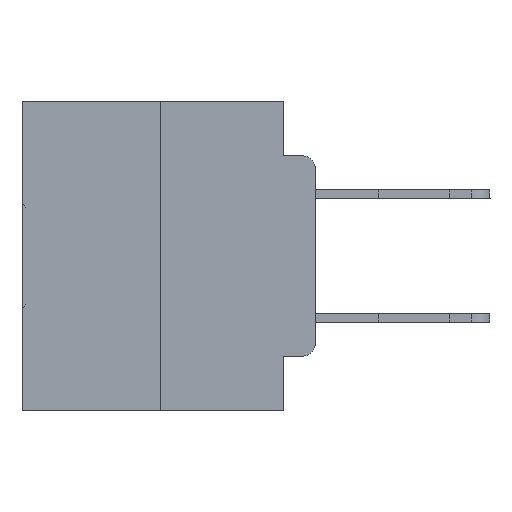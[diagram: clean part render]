
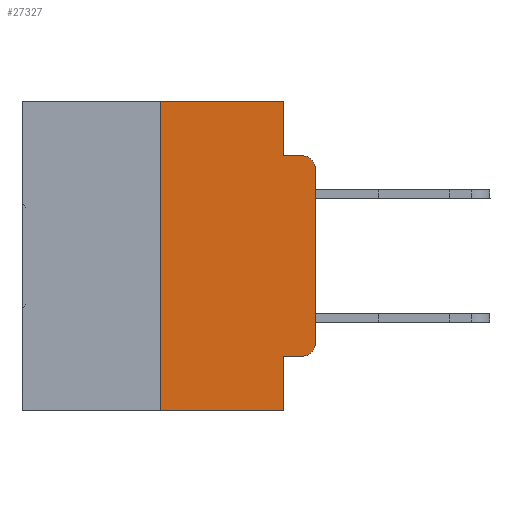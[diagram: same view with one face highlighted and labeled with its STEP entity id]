
A CAD part, left-side view. The second image highlights one B-rep face of the part: STEP entity #27327.
In plain terms, the highlighted planar face has unit normal (-1, 0, 0).
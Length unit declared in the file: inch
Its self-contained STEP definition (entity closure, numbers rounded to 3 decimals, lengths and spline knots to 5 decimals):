
#2213 = CARTESIAN_POINT ( 'NONE',  ( 0., 0.25, 0. ) ) ;
#2262 = VERTEX_POINT ( 'NONE', #5956 ) ;
#2728 = CARTESIAN_POINT ( 'NONE',  ( 0., 0.051, 0. ) ) ;
#3521 = VERTEX_POINT ( 'NONE', #10878 ) ;
#3592 = VERTEX_POINT ( 'NONE', #6604 ) ;
#4012 = ORIENTED_EDGE ( 'NONE', *, *, #5354, .F. ) ;
#4303 = DIRECTION ( 'NONE',  ( 0., -1., 0. ) ) ;
#4450 = VECTOR ( 'NONE', #5321, 39.37008 ) ;
#4704 = CARTESIAN_POINT ( 'NONE',  ( 0., 0.051, -0.0885 ) ) ;
#4944 = CARTESIAN_POINT ( 'NONE',  ( 0., 0.02, -0.0885 ) ) ;
#5089 = VERTEX_POINT ( 'NONE', #11363 ) ;
#5298 = EDGE_CURVE ( 'NONE', #19324, #2262, #17983, .T. ) ;
#5321 = DIRECTION ( 'NONE',  ( 0., 0., -1. ) ) ;
#5354 = EDGE_CURVE ( 'NONE', #12511, #17795, #28967, .T. ) ;
#5647 = PLANE ( 'NONE',  #28831 ) ;
#5956 = CARTESIAN_POINT ( 'NONE',  ( 0., 0.051, -0.5 ) ) ;
#6230 = ORIENTED_EDGE ( 'NONE', *, *, #12284, .F. ) ;
#6259 = ORIENTED_EDGE ( 'NONE', *, *, #5298, .T. ) ;
#6604 = CARTESIAN_POINT ( 'NONE',  ( 0., 0.02, -0.4115 ) ) ;
#6628 = DIRECTION ( 'NONE',  ( -1., 0., 0. ) ) ;
#6842 = VERTEX_POINT ( 'NONE', #19557 ) ;
#7045 = EDGE_CURVE ( 'NONE', #5089, #12511, #17865, .T. ) ;
#7647 = VECTOR ( 'NONE', #18603, 39.37008 ) ;
#8084 = VECTOR ( 'NONE', #4303, 39.37008 ) ;
#8150 = DIRECTION ( 'NONE',  ( 0., 0., -1. ) ) ;
#10613 = EDGE_LOOP ( 'NONE', ( #29082, #21397, #4012, #15840, #6230, #30624, #6259, #30481, #12213, #14582 ) ) ;
#10704 = VECTOR ( 'NONE', #24773, 39.37008 ) ;
#10878 = CARTESIAN_POINT ( 'NONE',  ( 0., 0., -0.1085 ) ) ;
#11234 = LINE ( 'NONE', #31539, #12017 ) ;
#11363 = CARTESIAN_POINT ( 'NONE',  ( 0., 0.051, 0. ) ) ;
#12017 = VECTOR ( 'NONE', #19038, 39.37008 ) ;
#12142 = EDGE_CURVE ( 'NONE', #6842, #2262, #21060, .T. ) ;
#12213 = ORIENTED_EDGE ( 'NONE', *, *, #20557, .T. ) ;
#12284 = EDGE_CURVE ( 'NONE', #32064, #5089, #11234, .T. ) ;
#12376 = DIRECTION ( 'NONE',  ( 0., -1., 0. ) ) ;
#12511 = VERTEX_POINT ( 'NONE', #4704 ) ;
#12925 = CARTESIAN_POINT ( 'NONE',  ( 0., 0.25, 0. ) ) ;
#13269 = LINE ( 'NONE', #30230, #25851 ) ;
#13841 = EDGE_CURVE ( 'NONE', #19324, #32064, #16252, .T. ) ;
#14211 = CIRCLE ( 'NONE', #20802, 0.02 ) ;
#14582 = ORIENTED_EDGE ( 'NONE', *, *, #15503, .T. ) ;
#14964 = DIRECTION ( 'NONE',  ( -1., 0., 0. ) ) ;
#15434 = DIRECTION ( 'NONE',  ( 0., 0., 1. ) ) ;
#15503 = EDGE_CURVE ( 'NONE', #3592, #26535, #14211, .T. ) ;
#15840 = ORIENTED_EDGE ( 'NONE', *, *, #7045, .F. ) ;
#16053 = CARTESIAN_POINT ( 'NONE',  ( 0., 0.051, 0. ) ) ;
#16252 = LINE ( 'NONE', #12925, #28836 ) ;
#17184 = VECTOR ( 'NONE', #12376, 39.37008 ) ;
#17795 = VERTEX_POINT ( 'NONE', #4944 ) ;
#17821 = EDGE_CURVE ( 'NONE', #26535, #3521, #13269, .T. ) ;
#17865 = LINE ( 'NONE', #2728, #4450 ) ;
#17983 = LINE ( 'NONE', #29927, #17184 ) ;
#18099 = CARTESIAN_POINT ( 'NONE',  ( 0., 0.473, 0. ) ) ;
#18603 = DIRECTION ( 'NONE',  ( 0., 0., -1. ) ) ;
#18857 = FACE_OUTER_BOUND ( 'NONE', #10613, .T. ) ;
#19038 = DIRECTION ( 'NONE',  ( 0., -1., 0. ) ) ;
#19324 = VERTEX_POINT ( 'NONE', #26350 ) ;
#19557 = CARTESIAN_POINT ( 'NONE',  ( 0., 0.051, -0.4115 ) ) ;
#20557 = EDGE_CURVE ( 'NONE', #6842, #3592, #30727, .T. ) ;
#20802 = AXIS2_PLACEMENT_3D ( 'NONE', #29999, #14964, #32491 ) ;
#21060 = LINE ( 'NONE', #16053, #7647 ) ;
#21397 = ORIENTED_EDGE ( 'NONE', *, *, #22882, .T. ) ;
#21741 = CARTESIAN_POINT ( 'NONE',  ( 0., 0.02, -0.1085 ) ) ;
#22209 = CARTESIAN_POINT ( 'NONE',  ( 0., 0.051, -0.4115 ) ) ;
#22795 = CIRCLE ( 'NONE', #31477, 0.02 ) ;
#22882 = EDGE_CURVE ( 'NONE', #3521, #17795, #22795, .T. ) ;
#23290 = DIRECTION ( 'NONE',  ( 1., 0., 0. ) ) ;
#24300 = DIRECTION ( 'NONE',  ( 0., 0., -1. ) ) ;
#24773 = DIRECTION ( 'NONE',  ( 0., -1., 0. ) ) ;
#25851 = VECTOR ( 'NONE', #32730, 39.37008 ) ;
#26350 = CARTESIAN_POINT ( 'NONE',  ( 0., 0.25, -0.5 ) ) ;
#26535 = VERTEX_POINT ( 'NONE', #29905 ) ;
#26990 = CARTESIAN_POINT ( 'NONE',  ( 0., 0.051, -0.0885 ) ) ;
#27327 = ADVANCED_FACE ( 'NONE', ( #18857 ), #5647, .F. ) ;
#28831 = AXIS2_PLACEMENT_3D ( 'NONE', #18099, #23290, #8150 ) ;
#28836 = VECTOR ( 'NONE', #15434, 39.37008 ) ;
#28967 = LINE ( 'NONE', #26990, #8084 ) ;
#29082 = ORIENTED_EDGE ( 'NONE', *, *, #17821, .T. ) ;
#29905 = CARTESIAN_POINT ( 'NONE',  ( 0., 0., -0.3915 ) ) ;
#29927 = CARTESIAN_POINT ( 'NONE',  ( 0., 0.473, -0.5 ) ) ;
#29999 = CARTESIAN_POINT ( 'NONE',  ( 0., 0.02, -0.3915 ) ) ;
#30230 = CARTESIAN_POINT ( 'NONE',  ( 0., 0., 0. ) ) ;
#30481 = ORIENTED_EDGE ( 'NONE', *, *, #12142, .F. ) ;
#30624 = ORIENTED_EDGE ( 'NONE', *, *, #13841, .F. ) ;
#30727 = LINE ( 'NONE', #22209, #10704 ) ;
#31477 = AXIS2_PLACEMENT_3D ( 'NONE', #21741, #6628, #24300 ) ;
#31539 = CARTESIAN_POINT ( 'NONE',  ( 0., 0.473, 0. ) ) ;
#32064 = VERTEX_POINT ( 'NONE', #2213 ) ;
#32491 = DIRECTION ( 'NONE',  ( 0., 0., -1. ) ) ;
#32730 = DIRECTION ( 'NONE',  ( 0., 0., 1. ) ) ;
